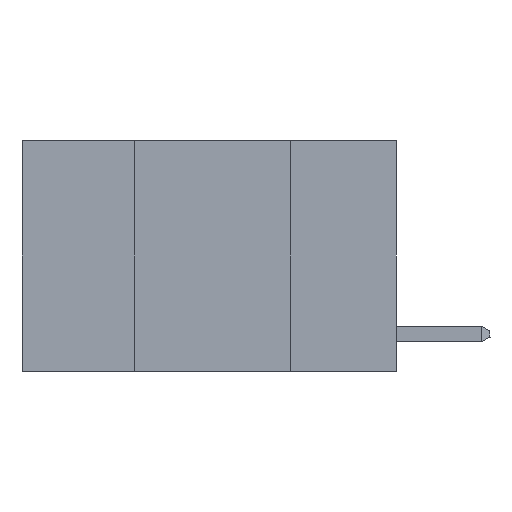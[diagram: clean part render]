
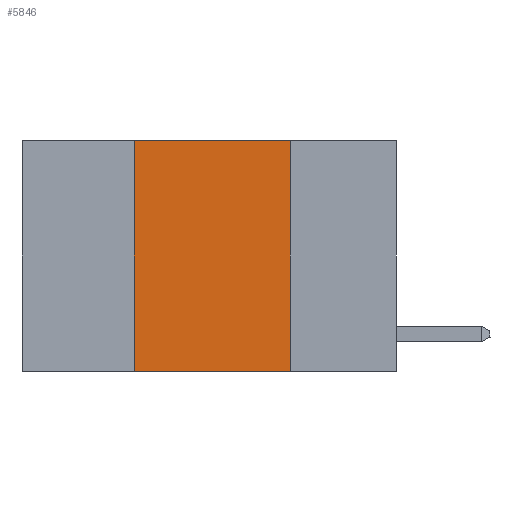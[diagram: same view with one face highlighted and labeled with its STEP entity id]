
A CAD part, left-side view. The second image highlights one B-rep face of the part: STEP entity #5846.
In plain terms, the highlighted planar face has unit normal (-1, 0, 0).
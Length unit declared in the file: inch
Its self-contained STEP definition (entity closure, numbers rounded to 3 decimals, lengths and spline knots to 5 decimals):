
#1139 = FACE_OUTER_BOUND ( 'NONE', #12380, .T. ) ;
#1246 = CARTESIAN_POINT ( 'NONE',  ( 0., 0.17, 0. ) ) ;
#1346 = EDGE_CURVE ( 'NONE', #6013, #5062, #3406, .T. ) ;
#1494 = AXIS2_PLACEMENT_3D ( 'NONE', #2055, #5121, #12458 ) ;
#1602 = ORIENTED_EDGE ( 'NONE', *, *, #10813, .T. ) ;
#2055 = CARTESIAN_POINT ( 'NONE',  ( 0., 0.6, 0. ) ) ;
#2668 = EDGE_CURVE ( 'NONE', #9269, #6013, #7883, .T. ) ;
#3148 = VERTEX_POINT ( 'NONE', #3805 ) ;
#3283 = DIRECTION ( 'NONE',  ( 0., 0., -1. ) ) ;
#3406 = LINE ( 'NONE', #7564, #8620 ) ;
#3805 = CARTESIAN_POINT ( 'NONE',  ( 0., 0.17, -0.37 ) ) ;
#3808 = ORIENTED_EDGE ( 'NONE', *, *, #4595, .F. ) ;
#3809 = ORIENTED_EDGE ( 'NONE', *, *, #2668, .F. ) ;
#3827 = LINE ( 'NONE', #13189, #12317 ) ;
#4167 = LINE ( 'NONE', #8350, #9806 ) ;
#4595 = EDGE_CURVE ( 'NONE', #5062, #3148, #4167, .T. ) ;
#4734 = DIRECTION ( 'NONE',  ( 0., 0., 1. ) ) ;
#5062 = VERTEX_POINT ( 'NONE', #1246 ) ;
#5121 = DIRECTION ( 'NONE',  ( 1., 0., 0. ) ) ;
#5766 = ORIENTED_EDGE ( 'NONE', *, *, #1346, .F. ) ;
#5846 = ADVANCED_FACE ( 'NONE', ( #1139 ), #11474, .F. ) ;
#6013 = VERTEX_POINT ( 'NONE', #12788 ) ;
#7564 = CARTESIAN_POINT ( 'NONE',  ( 0., 0.6, 0. ) ) ;
#7883 = LINE ( 'NONE', #9972, #8646 ) ;
#7913 = DIRECTION ( 'NONE',  ( 0., -1., 0. ) ) ;
#8350 = CARTESIAN_POINT ( 'NONE',  ( 0., 0.17, 0. ) ) ;
#8620 = VECTOR ( 'NONE', #7913, 39.37008 ) ;
#8646 = VECTOR ( 'NONE', #4734, 39.37008 ) ;
#9269 = VERTEX_POINT ( 'NONE', #12575 ) ;
#9806 = VECTOR ( 'NONE', #3283, 39.37008 ) ;
#9889 = DIRECTION ( 'NONE',  ( 0., -1., 0. ) ) ;
#9972 = CARTESIAN_POINT ( 'NONE',  ( 0., 0.42, 0. ) ) ;
#10813 = EDGE_CURVE ( 'NONE', #9269, #3148, #3827, .T. ) ;
#11474 = PLANE ( 'NONE',  #1494 ) ;
#12317 = VECTOR ( 'NONE', #9889, 39.37008 ) ;
#12380 = EDGE_LOOP ( 'NONE', ( #3808, #5766, #3809, #1602 ) ) ;
#12458 = DIRECTION ( 'NONE',  ( 0., 0., -1. ) ) ;
#12575 = CARTESIAN_POINT ( 'NONE',  ( 0., 0.42, -0.37 ) ) ;
#12788 = CARTESIAN_POINT ( 'NONE',  ( 0., 0.42, 0. ) ) ;
#13189 = CARTESIAN_POINT ( 'NONE',  ( 0., 0.6, -0.37 ) ) ;
